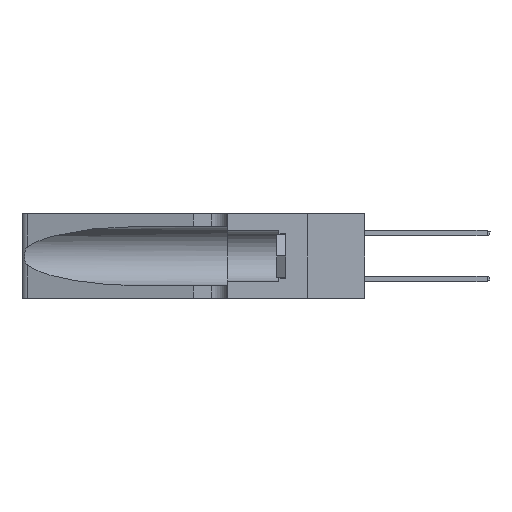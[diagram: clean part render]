
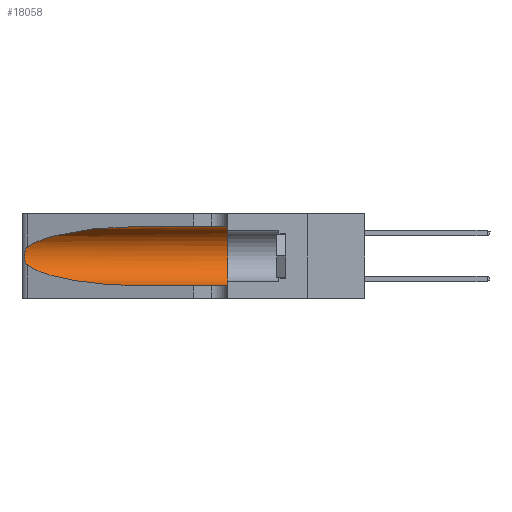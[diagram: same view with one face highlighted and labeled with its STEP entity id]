
A CAD part, left-side view. The second image highlights one B-rep face of the part: STEP entity #18058.
In plain terms, the highlighted cylindrical face has radius 3.308 mm (diameter 6.617 mm), a partial arc.
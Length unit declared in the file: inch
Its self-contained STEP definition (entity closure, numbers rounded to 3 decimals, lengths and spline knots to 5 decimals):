
#235 = ORIENTED_EDGE ( 'NONE', *, *, #17705, .F. ) ;
#648 = ORIENTED_EDGE ( 'NONE', *, *, #16696, .F. ) ;
#1842 = LINE ( 'NONE', #6121, #8946 ) ;
#1921 = CARTESIAN_POINT ( 'NONE',  ( 0.25555, 1.22994, 0.2215 ) ) ;
#2048 = EDGE_CURVE ( 'NONE', #9658, #33525, #36963, .T. ) ;
#2601 = CARTESIAN_POINT ( 'NONE',  ( 0.1305, 0.72297, 0.31525 ) ) ;
#2801 = DIRECTION ( 'NONE',  ( 0., -1., 0. ) ) ;
#3220 = CARTESIAN_POINT ( 'NONE',  ( 0.18966, 0.96281, 0.31525 ) ) ;
#4840 = CARTESIAN_POINT ( 'NONE',  ( 0.25854, 1.2359, 0.20912 ) ) ;
#5089 = CARTESIAN_POINT ( 'NONE',  ( 0.26017, 1.23833, 0.17102 ) ) ;
#5219 = CARTESIAN_POINT ( 'NONE',  ( 0.25856, 1.23593, 0.16098 ) ) ;
#5641 = ORIENTED_EDGE ( 'NONE', *, *, #2048, .T. ) ;
#5997 = B_SPLINE_CURVE_WITH_KNOTS ( 'NONE', 3,
 ( #34922, #1921, #37962, #35466, #4840, #11154, #29296, #35334, #5089, #5219, #8119, #23037, #25946, #10878 ),
 .UNSPECIFIED., .F., .F.,
 ( 4, 2, 2, 2, 2, 2, 4 ),
 ( 0., 0.00027, 0.00053, 0.00107, 0.0016, 0.00187, 0.00214 ),
 .UNSPECIFIED. ) ;
#6121 = CARTESIAN_POINT ( 'NONE',  ( 0.1305, 1.61858, 0.31525 ) ) ;
#7841 = VERTEX_POINT ( 'NONE', #17630 ) ;
#8119 = CARTESIAN_POINT ( 'NONE',  ( 0.25789, 1.23486, 0.15765 ) ) ;
#8946 = VECTOR ( 'NONE', #30201, 39.37008 ) ;
#9658 = VERTEX_POINT ( 'NONE', #26746 ) ;
#10878 = CARTESIAN_POINT ( 'NONE',  ( 0.25487, 1.22718, 0.14631 ) ) ;
#11154 = CARTESIAN_POINT ( 'NONE',  ( 0.26018, 1.23835, 0.19895 ) ) ;
#11320 = DIRECTION ( 'NONE',  ( 0., 1., 0. ) ) ;
#12416 = CARTESIAN_POINT ( 'NONE',  ( 0.2373, 1.15595, 0.28018 ) ) ;
#13972 =( BOUNDED_CURVE ( )  B_SPLINE_CURVE ( 3, ( #24703, #3220, #12416, #21542 ),
 .UNSPECIFIED., .F., .F. ) 
 B_SPLINE_CURVE_WITH_KNOTS ( ( 4, 4 ),
 ( 1.5708, 2.84003 ),
 .UNSPECIFIED. ) 
 CURVE ( )  GEOMETRIC_REPRESENTATION_ITEM ( )  RATIONAL_B_SPLINE_CURVE ( ( 1., 0.87, 0.87, 1. ) ) 
 REPRESENTATION_ITEM ( '' )  );
#14604 = CARTESIAN_POINT ( 'NONE',  ( 0.18966, 0.96281, 0.05475 ) ) ;
#14719 = CARTESIAN_POINT ( 'NONE',  ( 0.1305, 0.35, 0.31525 ) ) ;
#14847 = VERTEX_POINT ( 'NONE', #37139 ) ;
#15170 = DIRECTION ( 'NONE',  ( 0., -1., 0. ) ) ;
#15683 = ORIENTED_EDGE ( 'NONE', *, *, #26767, .T. ) ;
#16696 = EDGE_CURVE ( 'NONE', #38515, #14847, #17927, .T. ) ;
#16728 = EDGE_CURVE ( 'NONE', #34902, #7841, #13972, .T. ) ;
#17517 = CARTESIAN_POINT ( 'NONE',  ( 0.1305, 0.35, 0.185 ) ) ;
#17630 = CARTESIAN_POINT ( 'NONE',  ( 0.25487, 1.22718, 0.22369 ) ) ;
#17705 = EDGE_CURVE ( 'NONE', #34902, #38515, #1842, .T. ) ;
#17927 = CIRCLE ( 'NONE', #19514, 0.13025 ) ;
#18058 = ADVANCED_FACE ( 'NONE', ( #21635 ), #18781, .F. ) ;
#18781 = CYLINDRICAL_SURFACE ( 'NONE', #21952, 0.13025 ) ;
#19514 = AXIS2_PLACEMENT_3D ( 'NONE', #17517, #11320, #23480 ) ;
#20409 = CARTESIAN_POINT ( 'NONE',  ( 0.25487, 1.22718, 0.14631 ) ) ;
#21542 = CARTESIAN_POINT ( 'NONE',  ( 0.25487, 1.22718, 0.22369 ) ) ;
#21635 = FACE_OUTER_BOUND ( 'NONE', #32310, .T. ) ;
#21951 = ORIENTED_EDGE ( 'NONE', *, *, #16728, .T. ) ;
#21952 = AXIS2_PLACEMENT_3D ( 'NONE', #27615, #15170, #36816 ) ;
#23037 = CARTESIAN_POINT ( 'NONE',  ( 0.25639, 1.23186, 0.15144 ) ) ;
#23459 = CARTESIAN_POINT ( 'NONE',  ( 0.2373, 1.15595, 0.08982 ) ) ;
#23480 = DIRECTION ( 'NONE',  ( 0., 0., 1. ) ) ;
#23617 = LINE ( 'NONE', #26478, #24982 ) ;
#24703 = CARTESIAN_POINT ( 'NONE',  ( 0.1305, 0.72297, 0.31525 ) ) ;
#24982 = VECTOR ( 'NONE', #2801, 39.37008 ) ;
#25946 = CARTESIAN_POINT ( 'NONE',  ( 0.25555, 1.22993, 0.14849 ) ) ;
#26478 = CARTESIAN_POINT ( 'NONE',  ( 0.1305, 1.61858, 0.05475 ) ) ;
#26746 = CARTESIAN_POINT ( 'NONE',  ( 0.25487, 1.22718, 0.14631 ) ) ;
#26767 = EDGE_CURVE ( 'NONE', #7841, #9658, #5997, .T. ) ;
#27615 = CARTESIAN_POINT ( 'NONE',  ( 0.1305, 1.61858, 0.185 ) ) ;
#28542 = ORIENTED_EDGE ( 'NONE', *, *, #31916, .T. ) ;
#29296 = CARTESIAN_POINT ( 'NONE',  ( 0.26075, 1.23896, 0.19203 ) ) ;
#29857 = CARTESIAN_POINT ( 'NONE',  ( 0.1305, 0.72297, 0.05475 ) ) ;
#30201 = DIRECTION ( 'NONE',  ( 0., -1., 0. ) ) ;
#31916 = EDGE_CURVE ( 'NONE', #33525, #14847, #23617, .T. ) ;
#32310 = EDGE_LOOP ( 'NONE', ( #21951, #15683, #5641, #28542, #648, #235 ) ) ;
#33525 = VERTEX_POINT ( 'NONE', #35453 ) ;
#34902 = VERTEX_POINT ( 'NONE', #2601 ) ;
#34922 = CARTESIAN_POINT ( 'NONE',  ( 0.25487, 1.22718, 0.22369 ) ) ;
#35334 = CARTESIAN_POINT ( 'NONE',  ( 0.26075, 1.23896, 0.178 ) ) ;
#35453 = CARTESIAN_POINT ( 'NONE',  ( 0.1305, 0.72297, 0.05475 ) ) ;
#35466 = CARTESIAN_POINT ( 'NONE',  ( 0.25787, 1.23484, 0.2124 ) ) ;
#36816 = DIRECTION ( 'NONE',  ( 0., 0., -1. ) ) ;
#36963 =( BOUNDED_CURVE ( )  B_SPLINE_CURVE ( 3, ( #20409, #23459, #14604, #29857 ),
 .UNSPECIFIED., .F., .F. ) 
 B_SPLINE_CURVE_WITH_KNOTS ( ( 4, 4 ),
 ( 3.44316, 4.71239 ),
 .UNSPECIFIED. ) 
 CURVE ( )  GEOMETRIC_REPRESENTATION_ITEM ( )  RATIONAL_B_SPLINE_CURVE ( ( 1., 0.87, 0.87, 1. ) ) 
 REPRESENTATION_ITEM ( '' )  );
#37139 = CARTESIAN_POINT ( 'NONE',  ( 0.1305, 0.35, 0.05475 ) ) ;
#37962 = CARTESIAN_POINT ( 'NONE',  ( 0.25639, 1.23184, 0.21858 ) ) ;
#38515 = VERTEX_POINT ( 'NONE', #14719 ) ;
